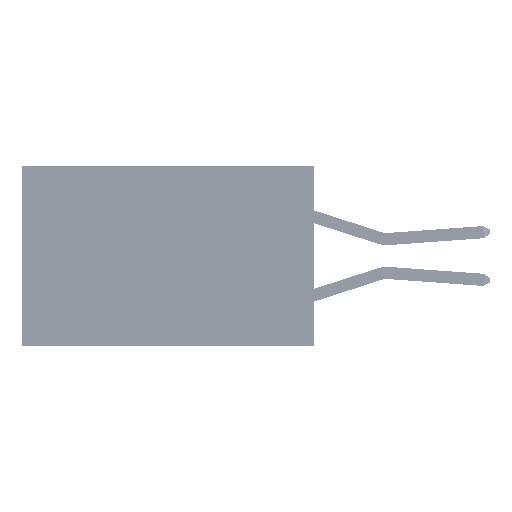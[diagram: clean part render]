
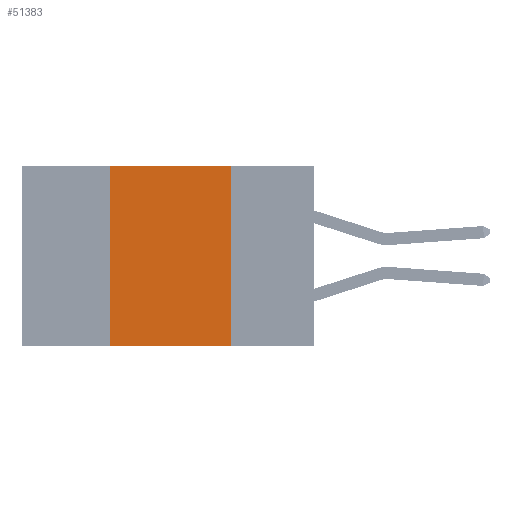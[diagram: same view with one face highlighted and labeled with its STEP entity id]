
A CAD part, left-side view. The second image highlights one B-rep face of the part: STEP entity #51383.
In plain terms, the highlighted planar face has unit normal (-1, 0, 0).
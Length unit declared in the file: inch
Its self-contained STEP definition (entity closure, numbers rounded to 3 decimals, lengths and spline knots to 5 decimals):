
#538 = CARTESIAN_POINT ( 'NONE',  ( 0., 0.17, -0.37 ) ) ;
#1335 = DIRECTION ( 'NONE',  ( 0., -1., 0. ) ) ;
#2443 = LINE ( 'NONE', #17957, #10944 ) ;
#4866 = LINE ( 'NONE', #12524, #10732 ) ;
#5260 = ORIENTED_EDGE ( 'NONE', *, *, #18113, .F. ) ;
#5287 = FACE_OUTER_BOUND ( 'NONE', #46469, .T. ) ;
#7141 = VERTEX_POINT ( 'NONE', #38468 ) ;
#7571 = ORIENTED_EDGE ( 'NONE', *, *, #21515, .F. ) ;
#10732 = VECTOR ( 'NONE', #25064, 39.37008 ) ;
#10944 = VECTOR ( 'NONE', #1335, 39.37008 ) ;
#12524 = CARTESIAN_POINT ( 'NONE',  ( 0., 0.42, 0. ) ) ;
#13952 = DIRECTION ( 'NONE',  ( 1., 0., 0. ) ) ;
#14307 = DIRECTION ( 'NONE',  ( 0., 0., -1. ) ) ;
#15778 = CARTESIAN_POINT ( 'NONE',  ( 0., 0.42, -0.37 ) ) ;
#17957 = CARTESIAN_POINT ( 'NONE',  ( 0., 0.6, 0. ) ) ;
#18113 = EDGE_CURVE ( 'NONE', #7141, #36180, #2443, .T. ) ;
#18160 = PLANE ( 'NONE',  #20388 ) ;
#18343 = CARTESIAN_POINT ( 'NONE',  ( 0., 0.6, 0. ) ) ;
#18653 = CARTESIAN_POINT ( 'NONE',  ( 0., 0.17, 0. ) ) ;
#20388 = AXIS2_PLACEMENT_3D ( 'NONE', #18343, #13952, #14307 ) ;
#21515 = EDGE_CURVE ( 'NONE', #24942, #7141, #4866, .T. ) ;
#24942 = VERTEX_POINT ( 'NONE', #15778 ) ;
#25064 = DIRECTION ( 'NONE',  ( 0., 0., 1. ) ) ;
#25739 = CARTESIAN_POINT ( 'NONE',  ( 0., 0.6, -0.37 ) ) ;
#26327 = EDGE_CURVE ( 'NONE', #24942, #28847, #44045, .T. ) ;
#27561 = ORIENTED_EDGE ( 'NONE', *, *, #26327, .T. ) ;
#28372 = EDGE_CURVE ( 'NONE', #36180, #28847, #36636, .T. ) ;
#28847 = VERTEX_POINT ( 'NONE', #538 ) ;
#36180 = VERTEX_POINT ( 'NONE', #53206 ) ;
#36636 = LINE ( 'NONE', #18653, #41261 ) ;
#38227 = VECTOR ( 'NONE', #42654, 39.37008 ) ;
#38468 = CARTESIAN_POINT ( 'NONE',  ( 0., 0.42, 0. ) ) ;
#41261 = VECTOR ( 'NONE', #51187, 39.37008 ) ;
#42654 = DIRECTION ( 'NONE',  ( 0., -1., 0. ) ) ;
#44045 = LINE ( 'NONE', #25739, #38227 ) ;
#46469 = EDGE_LOOP ( 'NONE', ( #48842, #5260, #7571, #27561 ) ) ;
#48842 = ORIENTED_EDGE ( 'NONE', *, *, #28372, .F. ) ;
#51187 = DIRECTION ( 'NONE',  ( 0., 0., -1. ) ) ;
#51383 = ADVANCED_FACE ( 'NONE', ( #5287 ), #18160, .F. ) ;
#53206 = CARTESIAN_POINT ( 'NONE',  ( 0., 0.17, 0. ) ) ;
